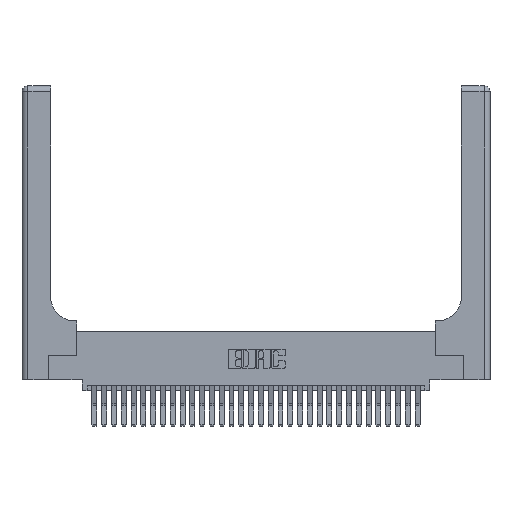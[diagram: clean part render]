
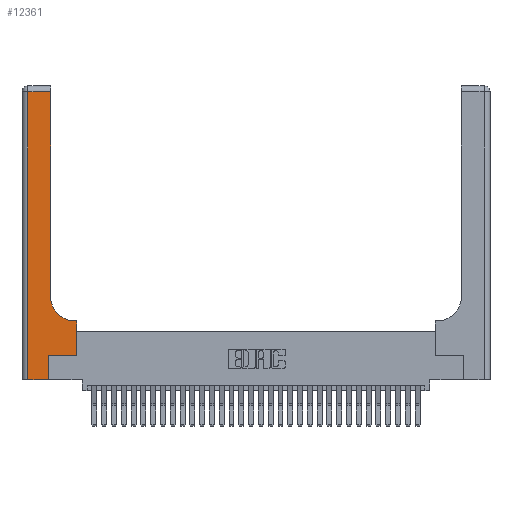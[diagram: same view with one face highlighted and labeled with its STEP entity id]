
A CAD part, top view. The second image highlights one B-rep face of the part: STEP entity #12361.
In plain terms, the highlighted planar face has unit normal (0, 0, 1).
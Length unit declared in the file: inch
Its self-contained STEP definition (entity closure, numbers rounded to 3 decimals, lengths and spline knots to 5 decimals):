
#42 = VERTEX_POINT ( 'NONE', #32563 ) ;
#456 = CARTESIAN_POINT ( 'NONE',  ( 0.5415, 0.85, 0.37 ) ) ;
#504 = DIRECTION ( 'NONE',  ( 0., 0., -1. ) ) ;
#793 = ORIENTED_EDGE ( 'NONE', *, *, #14627, .T. ) ;
#936 = VERTEX_POINT ( 'NONE', #22587 ) ;
#1563 = CARTESIAN_POINT ( 'NONE',  ( 0., 2.94, 0.37 ) ) ;
#1667 = ORIENTED_EDGE ( 'NONE', *, *, #28009, .T. ) ;
#2443 = ORIENTED_EDGE ( 'NONE', *, *, #18774, .T. ) ;
#3084 = DIRECTION ( 'NONE',  ( 1., 0., 0. ) ) ;
#3787 = EDGE_CURVE ( 'NONE', #42, #12625, #11608, .T. ) ;
#4865 = CARTESIAN_POINT ( 'NONE',  ( 0.269, 0.25, 0.37 ) ) ;
#5012 = DIRECTION ( 'NONE',  ( 0., 1., 0. ) ) ;
#5620 = VECTOR ( 'NONE', #14336, 39.37008 ) ;
#6741 = EDGE_LOOP ( 'NONE', ( #18958, #10867, #793, #24735, #20472, #22383, #1667, #31582, #2443 ) ) ;
#7057 = EDGE_CURVE ( 'NONE', #936, #11447, #28846, .T. ) ;
#7164 = VECTOR ( 'NONE', #7229, 39.37008 ) ;
#7229 = DIRECTION ( 'NONE',  ( 0., -1., 0. ) ) ;
#7654 = AXIS2_PLACEMENT_3D ( 'NONE', #16087, #504, #18676 ) ;
#8272 = PLANE ( 'NONE',  #7654 ) ;
#8450 = VERTEX_POINT ( 'NONE', #29467 ) ;
#8727 = EDGE_CURVE ( 'NONE', #12625, #26267, #30697, .T. ) ;
#8809 = CARTESIAN_POINT ( 'NONE',  ( 0., 0., 0.37 ) ) ;
#9274 = CARTESIAN_POINT ( 'NONE',  ( 0.2915, 2.94, 0.37 ) ) ;
#9963 = VECTOR ( 'NONE', #15601, 39.37008 ) ;
#10420 = DIRECTION ( 'NONE',  ( 0., 1., 0. ) ) ;
#10867 = ORIENTED_EDGE ( 'NONE', *, *, #8727, .T. ) ;
#11447 = VERTEX_POINT ( 'NONE', #22866 ) ;
#11608 = LINE ( 'NONE', #13037, #9963 ) ;
#12361 = ADVANCED_FACE ( 'NONE', ( #24548 ), #8272, .F. ) ;
#12625 = VERTEX_POINT ( 'NONE', #9274 ) ;
#13037 = CARTESIAN_POINT ( 'NONE',  ( 0.2915, 3., 0.37 ) ) ;
#13273 = EDGE_CURVE ( 'NONE', #22368, #29901, #19345, .T. ) ;
#14204 = VECTOR ( 'NONE', #30490, 39.37008 ) ;
#14336 = DIRECTION ( 'NONE',  ( -1., 0., 0. ) ) ;
#14627 = EDGE_CURVE ( 'NONE', #26267, #936, #20058, .T. ) ;
#15595 = CARTESIAN_POINT ( 'NONE',  ( 0.5585, 0.25, 0.37 ) ) ;
#15601 = DIRECTION ( 'NONE',  ( 0., 1., 0. ) ) ;
#15648 = CARTESIAN_POINT ( 'NONE',  ( 0.5585, 0.25, 0.37 ) ) ;
#16087 = CARTESIAN_POINT ( 'NONE',  ( 0., 3., 0.37 ) ) ;
#16444 = LINE ( 'NONE', #15595, #22412 ) ;
#16572 = CARTESIAN_POINT ( 'NONE',  ( 0.06, 2.94, 0.37 ) ) ;
#17048 = VECTOR ( 'NONE', #5012, 39.37008 ) ;
#17115 = DIRECTION ( 'NONE',  ( -1., 0., 0. ) ) ;
#17537 = CARTESIAN_POINT ( 'NONE',  ( 0.06, 3., 0.37 ) ) ;
#17618 = VERTEX_POINT ( 'NONE', #15648 ) ;
#18627 = DIRECTION ( 'NONE',  ( 0., 0., -1. ) ) ;
#18676 = DIRECTION ( 'NONE',  ( -1., 0., 0. ) ) ;
#18774 = EDGE_CURVE ( 'NONE', #29901, #42, #22633, .T. ) ;
#18958 = ORIENTED_EDGE ( 'NONE', *, *, #3787, .T. ) ;
#19153 = EDGE_CURVE ( 'NONE', #8450, #17618, #26152, .T. ) ;
#19345 = LINE ( 'NONE', #26991, #5620 ) ;
#20058 = LINE ( 'NONE', #17537, #7164 ) ;
#20472 = ORIENTED_EDGE ( 'NONE', *, *, #24211, .T. ) ;
#22003 = AXIS2_PLACEMENT_3D ( 'NONE', #456, #18627, #3084 ) ;
#22061 = CARTESIAN_POINT ( 'NONE',  ( 0.5585, 0.6, 0.37 ) ) ;
#22368 = VERTEX_POINT ( 'NONE', #22061 ) ;
#22383 = ORIENTED_EDGE ( 'NONE', *, *, #19153, .T. ) ;
#22412 = VECTOR ( 'NONE', #10420, 39.37008 ) ;
#22587 = CARTESIAN_POINT ( 'NONE',  ( 0.06, 0., 0.37 ) ) ;
#22633 = CIRCLE ( 'NONE', #22003, 0.25 ) ;
#22866 = CARTESIAN_POINT ( 'NONE',  ( 0.269, 0., 0.37 ) ) ;
#22935 = VECTOR ( 'NONE', #26690, 39.37008 ) ;
#24211 = EDGE_CURVE ( 'NONE', #11447, #8450, #32071, .T. ) ;
#24374 = CARTESIAN_POINT ( 'NONE',  ( 0.5415, 0.6, 0.37 ) ) ;
#24548 = FACE_OUTER_BOUND ( 'NONE', #6741, .T. ) ;
#24735 = ORIENTED_EDGE ( 'NONE', *, *, #7057, .T. ) ;
#24790 = VECTOR ( 'NONE', #17115, 39.37008 ) ;
#25588 = CARTESIAN_POINT ( 'NONE',  ( 0.269, 0., 0.37 ) ) ;
#26152 = LINE ( 'NONE', #4865, #14204 ) ;
#26267 = VERTEX_POINT ( 'NONE', #16572 ) ;
#26690 = DIRECTION ( 'NONE',  ( 1., 0., 0. ) ) ;
#26991 = CARTESIAN_POINT ( 'NONE',  ( 0.2915, 0.6, 0.37 ) ) ;
#28009 = EDGE_CURVE ( 'NONE', #17618, #22368, #16444, .T. ) ;
#28846 = LINE ( 'NONE', #8809, #22935 ) ;
#29467 = CARTESIAN_POINT ( 'NONE',  ( 0.269, 0.25, 0.37 ) ) ;
#29901 = VERTEX_POINT ( 'NONE', #24374 ) ;
#30490 = DIRECTION ( 'NONE',  ( 1., 0., 0. ) ) ;
#30697 = LINE ( 'NONE', #1563, #24790 ) ;
#31582 = ORIENTED_EDGE ( 'NONE', *, *, #13273, .T. ) ;
#32071 = LINE ( 'NONE', #25588, #17048 ) ;
#32563 = CARTESIAN_POINT ( 'NONE',  ( 0.2915, 0.85, 0.37 ) ) ;
